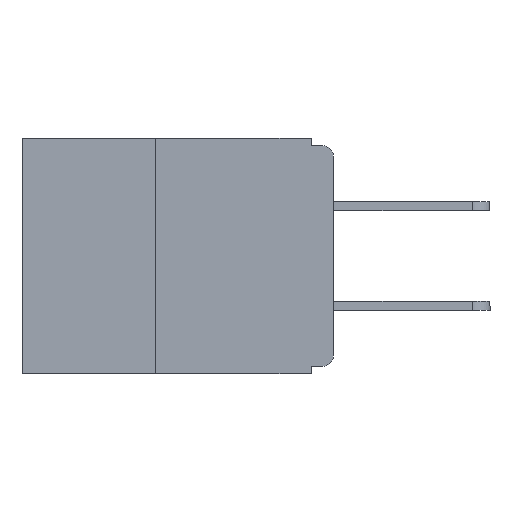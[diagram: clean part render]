
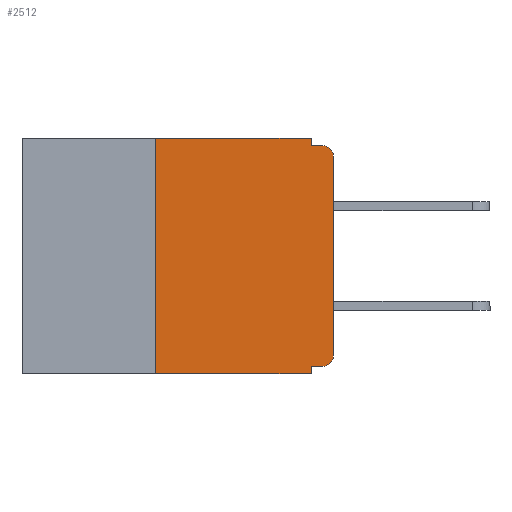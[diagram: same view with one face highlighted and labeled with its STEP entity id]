
A CAD part, left-side view. The second image highlights one B-rep face of the part: STEP entity #2512.
In plain terms, the highlighted planar face has unit normal (-1, 0, 0).
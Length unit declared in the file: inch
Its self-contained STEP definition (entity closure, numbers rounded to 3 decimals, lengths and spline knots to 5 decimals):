
#269 = AXIS2_PLACEMENT_3D ( 'NONE', #31644, #16769, #1487 ) ;
#388 = EDGE_CURVE ( 'NONE', #26613, #20853, #9878, .T. ) ;
#426 = EDGE_CURVE ( 'NONE', #17747, #7349, #15056, .T. ) ;
#1179 = VECTOR ( 'NONE', #16400, 39.37008 ) ;
#1487 = DIRECTION ( 'NONE',  ( 0., 0., -1. ) ) ;
#2279 = VERTEX_POINT ( 'NONE', #31097 ) ;
#2512 = ADVANCED_FACE ( 'NONE', ( #18496 ), #8389, .F. ) ;
#2985 = CARTESIAN_POINT ( 'NONE',  ( 0., 0., 0. ) ) ;
#3568 = VERTEX_POINT ( 'NONE', #31035 ) ;
#3585 = ORIENTED_EDGE ( 'NONE', *, *, #12895, .F. ) ;
#3839 = DIRECTION ( 'NONE',  ( 0., 0., 1. ) ) ;
#4461 = CARTESIAN_POINT ( 'NONE',  ( 0., 0.25, -0.33 ) ) ;
#5143 = EDGE_CURVE ( 'NONE', #3568, #12106, #21457, .T. ) ;
#5285 = CARTESIAN_POINT ( 'NONE',  ( 0., 0.437, -0.33 ) ) ;
#5358 = ORIENTED_EDGE ( 'NONE', *, *, #5584, .F. ) ;
#5584 = EDGE_CURVE ( 'NONE', #7349, #2279, #20607, .T. ) ;
#6136 = DIRECTION ( 'NONE',  ( 0., 0., -1. ) ) ;
#6582 = DIRECTION ( 'NONE',  ( 1., 0., 0. ) ) ;
#6945 = CARTESIAN_POINT ( 'NONE',  ( 0., 0.437, 0. ) ) ;
#7050 = ORIENTED_EDGE ( 'NONE', *, *, #14267, .F. ) ;
#7349 = VERTEX_POINT ( 'NONE', #21726 ) ;
#7679 = EDGE_CURVE ( 'NONE', #23267, #2279, #26924, .T. ) ;
#7849 = DIRECTION ( 'NONE',  ( 0., -1., 0. ) ) ;
#7852 = CARTESIAN_POINT ( 'NONE',  ( 0., 0.015, -0.32 ) ) ;
#7982 = EDGE_CURVE ( 'NONE', #12106, #20853, #24996, .T. ) ;
#8255 = VECTOR ( 'NONE', #26096, 39.37008 ) ;
#8389 = PLANE ( 'NONE',  #27493 ) ;
#8783 = VECTOR ( 'NONE', #3839, 39.37008 ) ;
#9479 = DIRECTION ( 'NONE',  ( 0., -1., 0. ) ) ;
#9536 = ORIENTED_EDGE ( 'NONE', *, *, #7982, .T. ) ;
#9878 = LINE ( 'NONE', #26117, #22508 ) ;
#10641 = VERTEX_POINT ( 'NONE', #10902 ) ;
#10902 = CARTESIAN_POINT ( 'NONE',  ( 0., 0.25, 0. ) ) ;
#11399 = LINE ( 'NONE', #27660, #24764 ) ;
#11436 = DIRECTION ( 'NONE',  ( -1., 0., 0. ) ) ;
#11557 = EDGE_CURVE ( 'NONE', #23267, #10641, #13418, .T. ) ;
#12106 = VERTEX_POINT ( 'NONE', #21843 ) ;
#12895 = EDGE_CURVE ( 'NONE', #10641, #20570, #19333, .T. ) ;
#13418 = LINE ( 'NONE', #4461, #19321 ) ;
#13595 = ORIENTED_EDGE ( 'NONE', *, *, #11557, .F. ) ;
#14267 = EDGE_CURVE ( 'NONE', #20570, #26613, #11399, .T. ) ;
#15056 = LINE ( 'NONE', #25995, #8255 ) ;
#16400 = DIRECTION ( 'NONE',  ( 0., 0., -1. ) ) ;
#16769 = DIRECTION ( 'NONE',  ( -1., 0., 0. ) ) ;
#16837 = AXIS2_PLACEMENT_3D ( 'NONE', #26434, #11436, #28902 ) ;
#17201 = DIRECTION ( 'NONE',  ( 0., 0., 1. ) ) ;
#17395 = CARTESIAN_POINT ( 'NONE',  ( 0., 0.031, -0.33 ) ) ;
#17747 = VERTEX_POINT ( 'NONE', #7852 ) ;
#18496 = FACE_OUTER_BOUND ( 'NONE', #21254, .T. ) ;
#19321 = VECTOR ( 'NONE', #17201, 39.37008 ) ;
#19333 = LINE ( 'NONE', #27215, #31756 ) ;
#19971 = CARTESIAN_POINT ( 'NONE',  ( 0., 0.031, 0. ) ) ;
#20570 = VERTEX_POINT ( 'NONE', #19971 ) ;
#20607 = LINE ( 'NONE', #17395, #1179 ) ;
#20853 = VERTEX_POINT ( 'NONE', #26073 ) ;
#21254 = EDGE_LOOP ( 'NONE', ( #27905, #9536, #30553, #7050, #3585, #13595, #21914, #5358, #27140, #27109 ) ) ;
#21457 = LINE ( 'NONE', #2985, #8783 ) ;
#21726 = CARTESIAN_POINT ( 'NONE',  ( 0., 0.031, -0.32 ) ) ;
#21843 = CARTESIAN_POINT ( 'NONE',  ( 0., 0., -0.025 ) ) ;
#21914 = ORIENTED_EDGE ( 'NONE', *, *, #7679, .T. ) ;
#22508 = VECTOR ( 'NONE', #9479, 39.37008 ) ;
#22914 = EDGE_CURVE ( 'NONE', #17747, #3568, #28820, .T. ) ;
#23267 = VERTEX_POINT ( 'NONE', #27723 ) ;
#24764 = VECTOR ( 'NONE', #25185, 39.37008 ) ;
#24996 = CIRCLE ( 'NONE', #269, 0.015 ) ;
#25185 = DIRECTION ( 'NONE',  ( 0., 0., -1. ) ) ;
#25995 = CARTESIAN_POINT ( 'NONE',  ( 0., 0., -0.32 ) ) ;
#26073 = CARTESIAN_POINT ( 'NONE',  ( 0., 0.015, -0.01 ) ) ;
#26096 = DIRECTION ( 'NONE',  ( 0., 1., 0. ) ) ;
#26117 = CARTESIAN_POINT ( 'NONE',  ( 0., 0., -0.01 ) ) ;
#26156 = VECTOR ( 'NONE', #7849, 39.37008 ) ;
#26434 = CARTESIAN_POINT ( 'NONE',  ( 0., 0.015, -0.305 ) ) ;
#26613 = VERTEX_POINT ( 'NONE', #26777 ) ;
#26777 = CARTESIAN_POINT ( 'NONE',  ( 0., 0.031, -0.01 ) ) ;
#26924 = LINE ( 'NONE', #5285, #26156 ) ;
#27109 = ORIENTED_EDGE ( 'NONE', *, *, #22914, .T. ) ;
#27140 = ORIENTED_EDGE ( 'NONE', *, *, #426, .F. ) ;
#27215 = CARTESIAN_POINT ( 'NONE',  ( 0., 0.437, 0. ) ) ;
#27493 = AXIS2_PLACEMENT_3D ( 'NONE', #6945, #6582, #6136 ) ;
#27660 = CARTESIAN_POINT ( 'NONE',  ( 0., 0.031, 0. ) ) ;
#27723 = CARTESIAN_POINT ( 'NONE',  ( 0., 0.25, -0.33 ) ) ;
#27905 = ORIENTED_EDGE ( 'NONE', *, *, #5143, .T. ) ;
#28820 = CIRCLE ( 'NONE', #16837, 0.015 ) ;
#28902 = DIRECTION ( 'NONE',  ( 0., 0., -1. ) ) ;
#29670 = DIRECTION ( 'NONE',  ( 0., -1., 0. ) ) ;
#30553 = ORIENTED_EDGE ( 'NONE', *, *, #388, .F. ) ;
#31035 = CARTESIAN_POINT ( 'NONE',  ( 0., 0., -0.305 ) ) ;
#31097 = CARTESIAN_POINT ( 'NONE',  ( 0., 0.031, -0.33 ) ) ;
#31644 = CARTESIAN_POINT ( 'NONE',  ( 0., 0.015, -0.025 ) ) ;
#31756 = VECTOR ( 'NONE', #29670, 39.37008 ) ;
